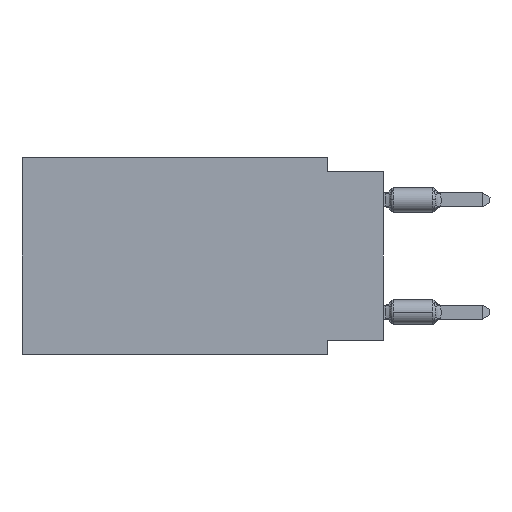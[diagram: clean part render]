
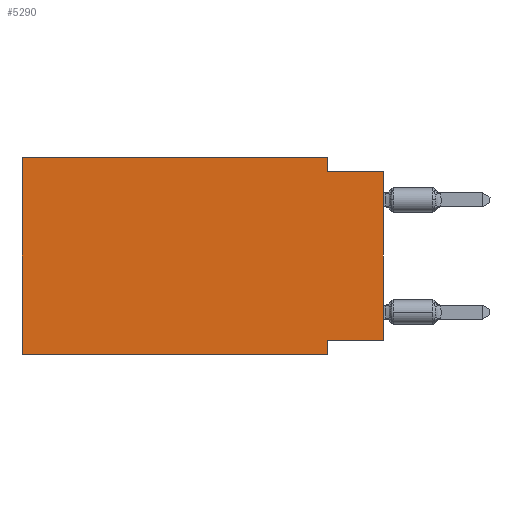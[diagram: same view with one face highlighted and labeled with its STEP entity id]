
A CAD part, left-side view. The second image highlights one B-rep face of the part: STEP entity #5290.
In plain terms, the highlighted planar face has unit normal (-1, 0, 0).
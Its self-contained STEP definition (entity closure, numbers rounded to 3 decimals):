
#237 = PLANE ( 'NONE',  #8798 ) ;
#573 = ORIENTED_EDGE ( 'NONE', *, *, #7714, .F. ) ;
#1247 = CARTESIAN_POINT ( 'NONE',  ( 0., 2.54, 0. ) ) ;
#1580 = VERTEX_POINT ( 'NONE', #2747 ) ;
#1887 = LINE ( 'NONE', #7934, #12011 ) ;
#2117 = EDGE_CURVE ( 'NONE', #2393, #2401, #1887, .T. ) ;
#2296 = VERTEX_POINT ( 'NONE', #17298 ) ;
#2393 = VERTEX_POINT ( 'NONE', #5834 ) ;
#2401 = VERTEX_POINT ( 'NONE', #13117 ) ;
#2632 = VERTEX_POINT ( 'NONE', #3640 ) ;
#2747 = CARTESIAN_POINT ( 'NONE',  ( 0., 2.54, -0.635 ) ) ;
#3058 = ORIENTED_EDGE ( 'NONE', *, *, #12060, .T. ) ;
#3138 = CARTESIAN_POINT ( 'NONE',  ( 0., 16.383, 0. ) ) ;
#3464 = EDGE_CURVE ( 'NONE', #1580, #2296, #6469, .T. ) ;
#3640 = CARTESIAN_POINT ( 'NONE',  ( 0., 2.54, -8.255 ) ) ;
#3686 = ORIENTED_EDGE ( 'NONE', *, *, #5265, .F. ) ;
#4552 = VECTOR ( 'NONE', #12833, 1000. ) ;
#4591 = LINE ( 'NONE', #4877, #10387 ) ;
#4877 = CARTESIAN_POINT ( 'NONE',  ( 0., 16.383, -8.89 ) ) ;
#4983 = DIRECTION ( 'NONE',  ( 0., -1., 0. ) ) ;
#5226 = VECTOR ( 'NONE', #18178, 1000. ) ;
#5265 = EDGE_CURVE ( 'NONE', #5570, #1580, #13290, .T. ) ;
#5290 = ADVANCED_FACE ( 'NONE', ( #9377 ), #237, .F. ) ;
#5570 = VERTEX_POINT ( 'NONE', #14580 ) ;
#5803 = VECTOR ( 'NONE', #5849, 1000. ) ;
#5834 = CARTESIAN_POINT ( 'NONE',  ( 0., 16.383, -8.89 ) ) ;
#5849 = DIRECTION ( 'NONE',  ( 0., 0., -1. ) ) ;
#5944 = ORIENTED_EDGE ( 'NONE', *, *, #18281, .F. ) ;
#6469 = LINE ( 'NONE', #7961, #15047 ) ;
#6655 = LINE ( 'NONE', #19013, #4552 ) ;
#7298 = DIRECTION ( 'NONE',  ( 0., 0., -1. ) ) ;
#7714 = EDGE_CURVE ( 'NONE', #17176, #2632, #18357, .T. ) ;
#7934 = CARTESIAN_POINT ( 'NONE',  ( 0., 16.383, 0. ) ) ;
#7961 = CARTESIAN_POINT ( 'NONE',  ( 0., 0., -0.635 ) ) ;
#8199 = EDGE_CURVE ( 'NONE', #2632, #11012, #18106, .T. ) ;
#8798 = AXIS2_PLACEMENT_3D ( 'NONE', #3138, #15182, #13767 ) ;
#9377 = FACE_OUTER_BOUND ( 'NONE', #11948, .T. ) ;
#9845 = EDGE_CURVE ( 'NONE', #17176, #2296, #6655, .T. ) ;
#10387 = VECTOR ( 'NONE', #10934, 1000. ) ;
#10934 = DIRECTION ( 'NONE',  ( 0., -1., 0. ) ) ;
#11012 = VERTEX_POINT ( 'NONE', #17011 ) ;
#11948 = EDGE_LOOP ( 'NONE', ( #19240, #19353, #3686, #5944, #16118, #3058, #15175, #573 ) ) ;
#12011 = VECTOR ( 'NONE', #18301, 1000. ) ;
#12060 = EDGE_CURVE ( 'NONE', #2393, #11012, #4591, .T. ) ;
#12470 = CARTESIAN_POINT ( 'NONE',  ( 0., 0., -8.255 ) ) ;
#12833 = DIRECTION ( 'NONE',  ( 0., 0., 1. ) ) ;
#13117 = CARTESIAN_POINT ( 'NONE',  ( 0., 16.383, 0. ) ) ;
#13230 = VECTOR ( 'NONE', #18546, 1000. ) ;
#13290 = LINE ( 'NONE', #1247, #17065 ) ;
#13315 = CARTESIAN_POINT ( 'NONE',  ( 0., 16.383, 0. ) ) ;
#13767 = DIRECTION ( 'NONE',  ( 0., 0., -1. ) ) ;
#14580 = CARTESIAN_POINT ( 'NONE',  ( 0., 2.54, 0. ) ) ;
#14999 = LINE ( 'NONE', #13315, #5226 ) ;
#15047 = VECTOR ( 'NONE', #4983, 1000. ) ;
#15122 = CARTESIAN_POINT ( 'NONE',  ( 0., 2.54, -8.89 ) ) ;
#15175 = ORIENTED_EDGE ( 'NONE', *, *, #8199, .F. ) ;
#15182 = DIRECTION ( 'NONE',  ( 1., 0., 0. ) ) ;
#15204 = CARTESIAN_POINT ( 'NONE',  ( 0., 0., -8.255 ) ) ;
#16118 = ORIENTED_EDGE ( 'NONE', *, *, #2117, .F. ) ;
#17011 = CARTESIAN_POINT ( 'NONE',  ( 0., 2.54, -8.89 ) ) ;
#17065 = VECTOR ( 'NONE', #7298, 1000. ) ;
#17176 = VERTEX_POINT ( 'NONE', #15204 ) ;
#17298 = CARTESIAN_POINT ( 'NONE',  ( 0., 0., -0.635 ) ) ;
#18106 = LINE ( 'NONE', #15122, #5803 ) ;
#18178 = DIRECTION ( 'NONE',  ( 0., -1., 0. ) ) ;
#18281 = EDGE_CURVE ( 'NONE', #2401, #5570, #14999, .T. ) ;
#18301 = DIRECTION ( 'NONE',  ( 0., 0., 1. ) ) ;
#18357 = LINE ( 'NONE', #12470, #13230 ) ;
#18546 = DIRECTION ( 'NONE',  ( 0., 1., 0. ) ) ;
#19013 = CARTESIAN_POINT ( 'NONE',  ( 0., 0., 0. ) ) ;
#19240 = ORIENTED_EDGE ( 'NONE', *, *, #9845, .T. ) ;
#19353 = ORIENTED_EDGE ( 'NONE', *, *, #3464, .F. ) ;
